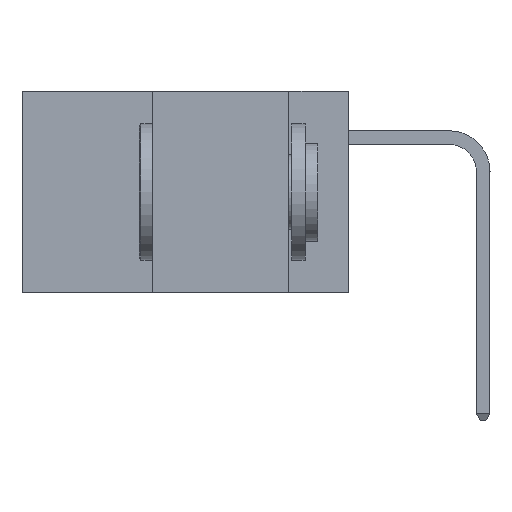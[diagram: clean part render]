
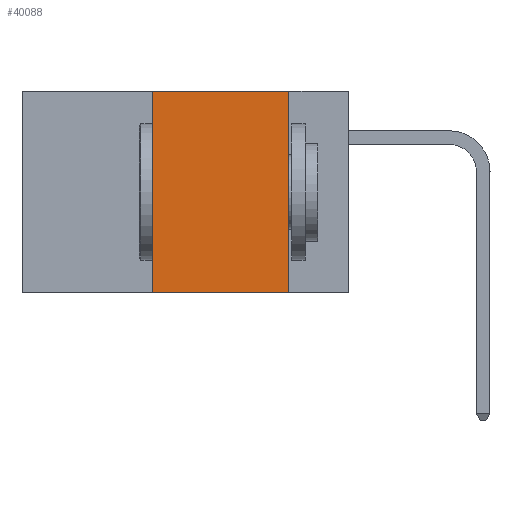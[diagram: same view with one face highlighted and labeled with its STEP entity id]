
A CAD part, left-side view. The second image highlights one B-rep face of the part: STEP entity #40088.
In plain terms, the highlighted planar face has unit normal (-1, 0, 0).
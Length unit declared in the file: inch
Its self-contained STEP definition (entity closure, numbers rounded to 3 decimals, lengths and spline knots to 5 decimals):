
#274 = DIRECTION ( 'NONE',  ( 1., 0., 0. ) ) ;
#1948 = VERTEX_POINT ( 'NONE', #40712 ) ;
#2069 = CARTESIAN_POINT ( 'NONE',  ( 0., 0.6, 0. ) ) ;
#2242 = CARTESIAN_POINT ( 'NONE',  ( 0., 0.36, 0. ) ) ;
#2273 = VERTEX_POINT ( 'NONE', #35428 ) ;
#4056 = CARTESIAN_POINT ( 'NONE',  ( 0., 0.6, -0.37 ) ) ;
#4209 = DIRECTION ( 'NONE',  ( 0., -1., 0. ) ) ;
#5508 = DIRECTION ( 'NONE',  ( 0., -1., 0. ) ) ;
#6045 = CARTESIAN_POINT ( 'NONE',  ( 0., 0.11, 0. ) ) ;
#8120 = EDGE_CURVE ( 'NONE', #26399, #2273, #37040, .T. ) ;
#10946 = FACE_OUTER_BOUND ( 'NONE', #24556, .T. ) ;
#11029 = VECTOR ( 'NONE', #26489, 39.37008 ) ;
#13156 = LINE ( 'NONE', #6045, #11029 ) ;
#13645 = EDGE_CURVE ( 'NONE', #34403, #1948, #32344, .T. ) ;
#13847 = ORIENTED_EDGE ( 'NONE', *, *, #39240, .F. ) ;
#14401 = ORIENTED_EDGE ( 'NONE', *, *, #24701, .F. ) ;
#20764 = DIRECTION ( 'NONE',  ( 0., 0., 1. ) ) ;
#21516 = LINE ( 'NONE', #41133, #39579 ) ;
#22256 = VECTOR ( 'NONE', #4209, 39.37008 ) ;
#24223 = DIRECTION ( 'NONE',  ( 0., 0., -1. ) ) ;
#24556 = EDGE_LOOP ( 'NONE', ( #13847, #28742, #14401, #35158 ) ) ;
#24701 = EDGE_CURVE ( 'NONE', #34403, #26399, #21516, .T. ) ;
#26399 = VERTEX_POINT ( 'NONE', #2242 ) ;
#26489 = DIRECTION ( 'NONE',  ( 0., 0., -1. ) ) ;
#28742 = ORIENTED_EDGE ( 'NONE', *, *, #8120, .F. ) ;
#29096 = VECTOR ( 'NONE', #5508, 39.37008 ) ;
#32344 = LINE ( 'NONE', #4056, #22256 ) ;
#34403 = VERTEX_POINT ( 'NONE', #40930 ) ;
#35158 = ORIENTED_EDGE ( 'NONE', *, *, #13645, .T. ) ;
#35428 = CARTESIAN_POINT ( 'NONE',  ( 0., 0.11, 0. ) ) ;
#37040 = LINE ( 'NONE', #2069, #29096 ) ;
#37659 = CARTESIAN_POINT ( 'NONE',  ( 0., 0.6, 0. ) ) ;
#39240 = EDGE_CURVE ( 'NONE', #2273, #1948, #13156, .T. ) ;
#39579 = VECTOR ( 'NONE', #20764, 39.37008 ) ;
#40088 = ADVANCED_FACE ( 'NONE', ( #10946 ), #41150, .F. ) ;
#40712 = CARTESIAN_POINT ( 'NONE',  ( 0., 0.11, -0.37 ) ) ;
#40930 = CARTESIAN_POINT ( 'NONE',  ( 0., 0.36, -0.37 ) ) ;
#41133 = CARTESIAN_POINT ( 'NONE',  ( 0., 0.36, 0. ) ) ;
#41150 = PLANE ( 'NONE',  #41437 ) ;
#41437 = AXIS2_PLACEMENT_3D ( 'NONE', #37659, #274, #24223 ) ;
